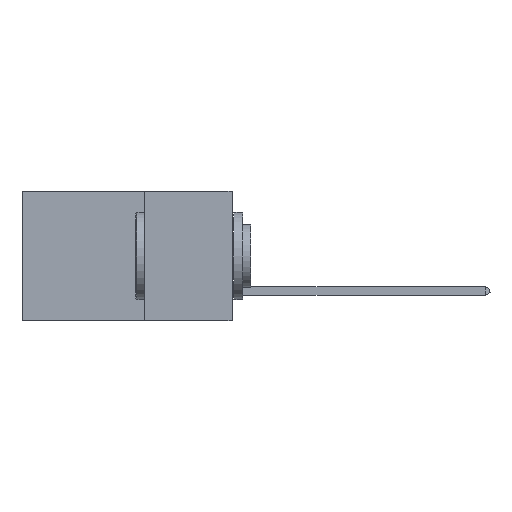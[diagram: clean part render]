
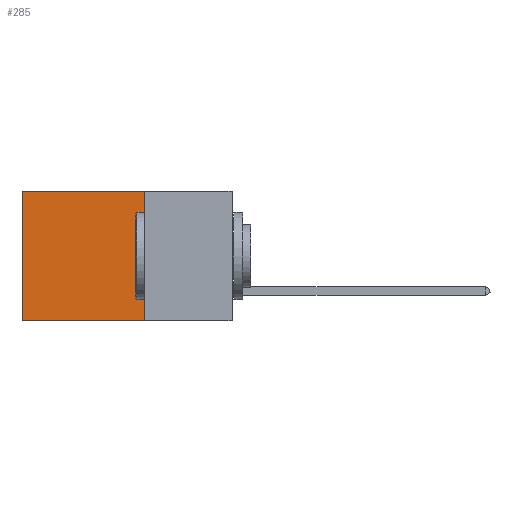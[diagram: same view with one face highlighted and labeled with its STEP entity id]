
A CAD part, left-side view. The second image highlights one B-rep face of the part: STEP entity #285.
In plain terms, the highlighted planar face has unit normal (-1, 0, 0).
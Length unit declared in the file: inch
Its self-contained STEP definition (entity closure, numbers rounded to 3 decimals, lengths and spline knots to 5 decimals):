
#285 = ADVANCED_FACE ( 'NONE', ( #23526 ), #367, .F. ) ;
#367 = PLANE ( 'NONE',  #2867 ) ;
#556 = EDGE_CURVE ( 'NONE', #19527, #27876, #29859, .T. ) ;
#839 = ORIENTED_EDGE ( 'NONE', *, *, #5984, .T. ) ;
#1161 = VECTOR ( 'NONE', #16756, 39.37008 ) ;
#2867 = AXIS2_PLACEMENT_3D ( 'NONE', #22975, #17982, #15456 ) ;
#3662 = VECTOR ( 'NONE', #6805, 39.37008 ) ;
#5984 = EDGE_CURVE ( 'NONE', #23208, #27876, #25363, .T. ) ;
#6805 = DIRECTION ( 'NONE',  ( 0., 1., 0. ) ) ;
#8748 = VERTEX_POINT ( 'NONE', #25338 ) ;
#11972 = CARTESIAN_POINT ( 'NONE',  ( 0.2875, 0.25, 0. ) ) ;
#12547 = ORIENTED_EDGE ( 'NONE', *, *, #19022, .F. ) ;
#13350 = DIRECTION ( 'NONE',  ( 0., 0., -1. ) ) ;
#14573 = EDGE_LOOP ( 'NONE', ( #839, #31440, #12547, #14609 ) ) ;
#14609 = ORIENTED_EDGE ( 'NONE', *, *, #23868, .T. ) ;
#15456 = DIRECTION ( 'NONE',  ( 0., 0., -1. ) ) ;
#16524 = CARTESIAN_POINT ( 'NONE',  ( 0.2875, 0.25, -0.37 ) ) ;
#16756 = DIRECTION ( 'NONE',  ( 0., 0., -1. ) ) ;
#17982 = DIRECTION ( 'NONE',  ( 1., 0., 0. ) ) ;
#19022 = EDGE_CURVE ( 'NONE', #8748, #19527, #21913, .T. ) ;
#19281 = CARTESIAN_POINT ( 'NONE',  ( 0.2875, 0.6, 0. ) ) ;
#19527 = VERTEX_POINT ( 'NONE', #25814 ) ;
#21913 = LINE ( 'NONE', #28526, #27110 ) ;
#22331 = DIRECTION ( 'NONE',  ( 0., 1., 0. ) ) ;
#22975 = CARTESIAN_POINT ( 'NONE',  ( 0.2875, 0.25, 0. ) ) ;
#23208 = VERTEX_POINT ( 'NONE', #19281 ) ;
#23526 = FACE_OUTER_BOUND ( 'NONE', #14573, .T. ) ;
#23868 = EDGE_CURVE ( 'NONE', #8748, #23208, #24546, .T. ) ;
#24546 = LINE ( 'NONE', #11972, #28500 ) ;
#25338 = CARTESIAN_POINT ( 'NONE',  ( 0.2875, 0.25, 0. ) ) ;
#25363 = LINE ( 'NONE', #26643, #1161 ) ;
#25814 = CARTESIAN_POINT ( 'NONE',  ( 0.2875, 0.25, -0.37 ) ) ;
#26643 = CARTESIAN_POINT ( 'NONE',  ( 0.2875, 0.6, 0. ) ) ;
#27110 = VECTOR ( 'NONE', #13350, 39.37008 ) ;
#27876 = VERTEX_POINT ( 'NONE', #32463 ) ;
#28500 = VECTOR ( 'NONE', #22331, 39.37008 ) ;
#28526 = CARTESIAN_POINT ( 'NONE',  ( 0.2875, 0.25, 0. ) ) ;
#29859 = LINE ( 'NONE', #16524, #3662 ) ;
#31440 = ORIENTED_EDGE ( 'NONE', *, *, #556, .F. ) ;
#32463 = CARTESIAN_POINT ( 'NONE',  ( 0.2875, 0.6, -0.37 ) ) ;
